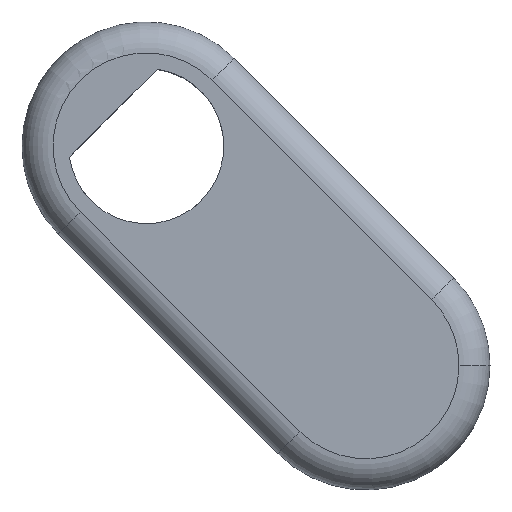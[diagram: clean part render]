
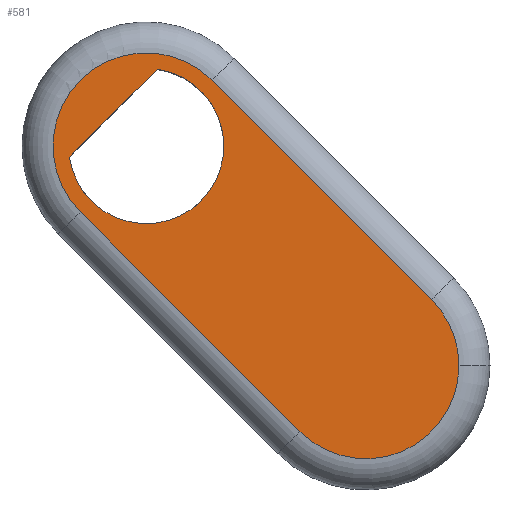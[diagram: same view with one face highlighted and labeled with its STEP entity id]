
A CAD part, top view. The second image highlights one B-rep face of the part: STEP entity #581.
In plain terms, the highlighted planar face has unit normal (0, 0, 1).
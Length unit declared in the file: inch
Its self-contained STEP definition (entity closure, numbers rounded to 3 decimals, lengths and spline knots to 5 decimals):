
#27 = DIRECTION ( 'NONE',  ( 0., 0., 1. ) ) ;
#40 = FACE_BOUND ( 'NONE', #627, .T. ) ;
#50 = CIRCLE ( 'NONE', #345, 0.11811 ) ;
#62 = LINE ( 'NONE', #645, #491 ) ;
#72 = ORIENTED_EDGE ( 'NONE', *, *, #459, .F. ) ;
#87 = CARTESIAN_POINT ( 'NONE',  ( 0., 0., 0.29528 ) ) ;
#99 = CARTESIAN_POINT ( 'NONE',  ( 0., 0., 0.29528 ) ) ;
#128 = VERTEX_POINT ( 'NONE', #582 ) ;
#145 = VERTEX_POINT ( 'NONE', #483 ) ;
#148 = DIRECTION ( 'NONE',  ( -1., 0., 0. ) ) ;
#150 = CARTESIAN_POINT ( 'NONE',  ( 0.3965, -0.27839, 0.29528 ) ) ;
#153 = CARTESIAN_POINT ( 'NONE',  ( 0., 0., 0.29528 ) ) ;
#169 = FACE_OUTER_BOUND ( 'NONE', #282, .T. ) ;
#173 = VECTOR ( 'NONE', #383, 39.37008 ) ;
#182 = ORIENTED_EDGE ( 'NONE', *, *, #428, .T. ) ;
#185 = CARTESIAN_POINT ( 'NONE',  ( 0.01392, 0.09744, 0.29528 ) ) ;
#186 = DIRECTION ( 'NONE',  ( 0., 0., 1. ) ) ;
#188 = CARTESIAN_POINT ( 'NONE',  ( 0.27839, -0.27839, 0.29528 ) ) ;
#191 = LINE ( 'NONE', #648, #173 ) ;
#196 = DIRECTION ( 'NONE',  ( -0.707, -0.707, 0. ) ) ;
#238 = VERTEX_POINT ( 'NONE', #248 ) ;
#245 = AXIS2_PLACEMENT_3D ( 'NONE', #87, #186, #593 ) ;
#246 = CARTESIAN_POINT ( 'NONE',  ( 0.27839, -0.27839, 0.29528 ) ) ;
#248 = CARTESIAN_POINT ( 'NONE',  ( 0.36191, -0.19487, 0.29528 ) ) ;
#249 = DIRECTION ( 'NONE',  ( 1., 0., 0. ) ) ;
#259 = DIRECTION ( 'NONE',  ( -0.707, 0.707, 0. ) ) ;
#262 = ORIENTED_EDGE ( 'NONE', *, *, #422, .T. ) ;
#282 = EDGE_LOOP ( 'NONE', ( #262, #182, #554, #623, #562 ) ) ;
#298 = VERTEX_POINT ( 'NONE', #312 ) ;
#305 = DIRECTION ( 'NONE',  ( 1., 0., 0. ) ) ;
#312 = CARTESIAN_POINT ( 'NONE',  ( -0.09744, -0.01392, 0.29528 ) ) ;
#314 = CARTESIAN_POINT ( 'NONE',  ( -0.04176, 0.04176, 0.29528 ) ) ;
#329 = CIRCLE ( 'NONE', #373, 0.11811 ) ;
#335 = AXIS2_PLACEMENT_3D ( 'NONE', #99, #496, #148 ) ;
#345 = AXIS2_PLACEMENT_3D ( 'NONE', #188, #595, #249 ) ;
#347 = CIRCLE ( 'NONE', #353, 0.11811 ) ;
#353 = AXIS2_PLACEMENT_3D ( 'NONE', #153, #27, #546 ) ;
#373 = AXIS2_PLACEMENT_3D ( 'NONE', #246, #637, #305 ) ;
#377 = ORIENTED_EDGE ( 'NONE', *, *, #454, .F. ) ;
#383 = DIRECTION ( 'NONE',  ( 0.707, -0.707, 0. ) ) ;
#420 = VERTEX_POINT ( 'NONE', #150 ) ;
#422 = EDGE_CURVE ( 'NONE', #238, #145, #62, .T. ) ;
#424 = VERTEX_POINT ( 'NONE', #605 ) ;
#426 = EDGE_CURVE ( 'NONE', #424, #128, #191, .T. ) ;
#428 = EDGE_CURVE ( 'NONE', #145, #424, #347, .T. ) ;
#434 = EDGE_CURVE ( 'NONE', #420, #238, #329, .T. ) ;
#437 = VECTOR ( 'NONE', #196, 39.37008 ) ;
#441 = EDGE_CURVE ( 'NONE', #128, #420, #50, .T. ) ;
#443 = VERTEX_POINT ( 'NONE', #185 ) ;
#454 = EDGE_CURVE ( 'NONE', #298, #443, #455, .T. ) ;
#455 = CIRCLE ( 'NONE', #335, 0.09843 ) ;
#459 = EDGE_CURVE ( 'NONE', #443, #298, #583, .T. ) ;
#483 = CARTESIAN_POINT ( 'NONE',  ( 0.08352, 0.08352, 0.29528 ) ) ;
#491 = VECTOR ( 'NONE', #259, 39.37008 ) ;
#496 = DIRECTION ( 'NONE',  ( 0., 0., 1. ) ) ;
#546 = DIRECTION ( 'NONE',  ( 1., 0., 0. ) ) ;
#548 = PLANE ( 'NONE',  #245 ) ;
#554 = ORIENTED_EDGE ( 'NONE', *, *, #426, .T. ) ;
#562 = ORIENTED_EDGE ( 'NONE', *, *, #434, .T. ) ;
#581 = ADVANCED_FACE ( 'NONE', ( #169, #40 ), #548, .T. ) ;
#582 = CARTESIAN_POINT ( 'NONE',  ( 0.19487, -0.36191, 0.29528 ) ) ;
#583 = LINE ( 'NONE', #314, #437 ) ;
#593 = DIRECTION ( 'NONE',  ( 1., 0., 0. ) ) ;
#595 = DIRECTION ( 'NONE',  ( 0., 0., 1. ) ) ;
#605 = CARTESIAN_POINT ( 'NONE',  ( -0.08352, -0.08352, 0.29528 ) ) ;
#623 = ORIENTED_EDGE ( 'NONE', *, *, #441, .T. ) ;
#627 = EDGE_LOOP ( 'NONE', ( #72, #377 ) ) ;
#637 = DIRECTION ( 'NONE',  ( 0., 0., 1. ) ) ;
#645 = CARTESIAN_POINT ( 'NONE',  ( 0.08352, 0.08352, 0.29528 ) ) ;
#648 = CARTESIAN_POINT ( 'NONE',  ( -0.08352, -0.08352, 0.29528 ) ) ;
